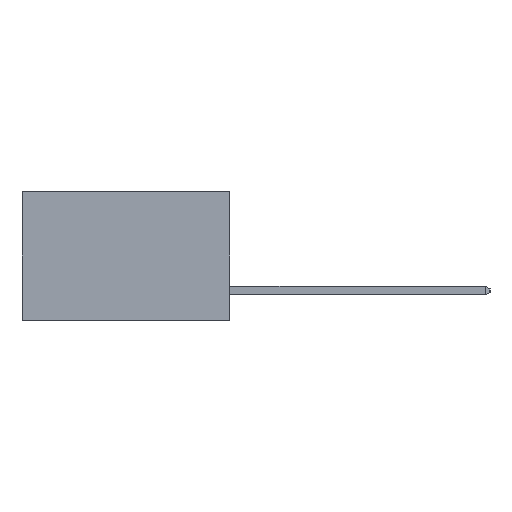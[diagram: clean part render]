
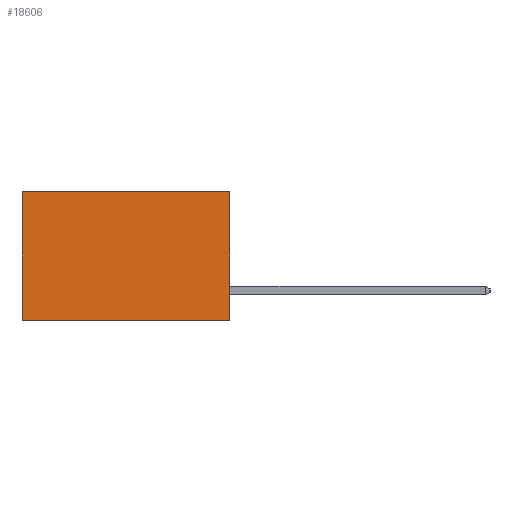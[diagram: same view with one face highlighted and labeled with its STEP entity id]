
A CAD part, left-side view. The second image highlights one B-rep face of the part: STEP entity #18606.
In plain terms, the highlighted planar face has unit normal (-1, 0, 0).
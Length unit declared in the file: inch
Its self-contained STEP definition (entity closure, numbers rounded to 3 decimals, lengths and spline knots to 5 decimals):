
#98 = VERTEX_POINT ( 'NONE', #10706 ) ;
#391 = ORIENTED_EDGE ( 'NONE', *, *, #18391, .T. ) ;
#981 = VERTEX_POINT ( 'NONE', #9156 ) ;
#1995 = DIRECTION ( 'NONE',  ( 0., 1., 0. ) ) ;
#2746 = LINE ( 'NONE', #7809, #6780 ) ;
#4034 = DIRECTION ( 'NONE',  ( 0., 1., 0. ) ) ;
#4271 = CARTESIAN_POINT ( 'NONE',  ( 0.298, 0., 0. ) ) ;
#4968 = CARTESIAN_POINT ( 'NONE',  ( 0.298, 0., 0. ) ) ;
#5492 = VERTEX_POINT ( 'NONE', #20970 ) ;
#5818 = CARTESIAN_POINT ( 'NONE',  ( 0.298, 0., 0. ) ) ;
#6541 = EDGE_CURVE ( 'NONE', #15323, #981, #20170, .T. ) ;
#6677 = DIRECTION ( 'NONE',  ( 0., 0., -1. ) ) ;
#6780 = VECTOR ( 'NONE', #20933, 39.37008 ) ;
#6845 = EDGE_CURVE ( 'NONE', #15323, #5492, #10188, .T. ) ;
#7809 = CARTESIAN_POINT ( 'NONE',  ( 0.298, 0.6, 0. ) ) ;
#8336 = PLANE ( 'NONE',  #14936 ) ;
#9156 = CARTESIAN_POINT ( 'NONE',  ( 0.298, 0.6, 0. ) ) ;
#10188 = LINE ( 'NONE', #12641, #18410 ) ;
#10706 = CARTESIAN_POINT ( 'NONE',  ( 0.298, 0.6, -0.37 ) ) ;
#10872 = CARTESIAN_POINT ( 'NONE',  ( 0.298, 0., -0.37 ) ) ;
#11701 = ORIENTED_EDGE ( 'NONE', *, *, #6541, .T. ) ;
#12641 = CARTESIAN_POINT ( 'NONE',  ( 0.298, 0., 0. ) ) ;
#12677 = VECTOR ( 'NONE', #4034, 39.37008 ) ;
#14936 = AXIS2_PLACEMENT_3D ( 'NONE', #4968, #16621, #6677 ) ;
#15241 = ORIENTED_EDGE ( 'NONE', *, *, #15762, .F. ) ;
#15323 = VERTEX_POINT ( 'NONE', #4271 ) ;
#15762 = EDGE_CURVE ( 'NONE', #5492, #98, #18012, .T. ) ;
#16621 = DIRECTION ( 'NONE',  ( 1., 0., 0. ) ) ;
#16920 = DIRECTION ( 'NONE',  ( 0., 0., -1. ) ) ;
#17089 = EDGE_LOOP ( 'NONE', ( #391, #15241, #18700, #11701 ) ) ;
#18012 = LINE ( 'NONE', #10872, #12677 ) ;
#18391 = EDGE_CURVE ( 'NONE', #981, #98, #2746, .T. ) ;
#18410 = VECTOR ( 'NONE', #16920, 39.37008 ) ;
#18606 = ADVANCED_FACE ( 'NONE', ( #19186 ), #8336, .F. ) ;
#18700 = ORIENTED_EDGE ( 'NONE', *, *, #6845, .F. ) ;
#19186 = FACE_OUTER_BOUND ( 'NONE', #17089, .T. ) ;
#20170 = LINE ( 'NONE', #5818, #20663 ) ;
#20663 = VECTOR ( 'NONE', #1995, 39.37008 ) ;
#20933 = DIRECTION ( 'NONE',  ( 0., 0., -1. ) ) ;
#20970 = CARTESIAN_POINT ( 'NONE',  ( 0.298, 0., -0.37 ) ) ;
